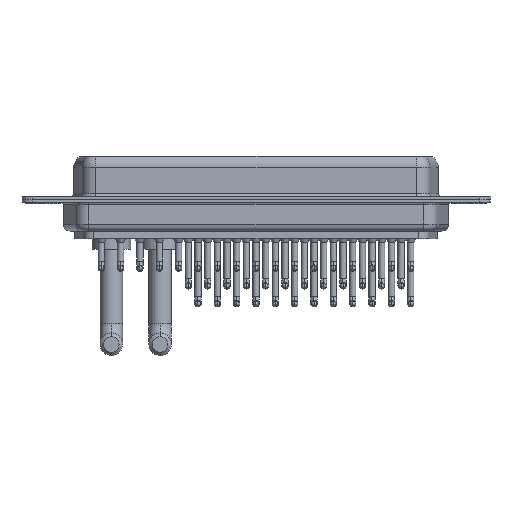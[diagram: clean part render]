
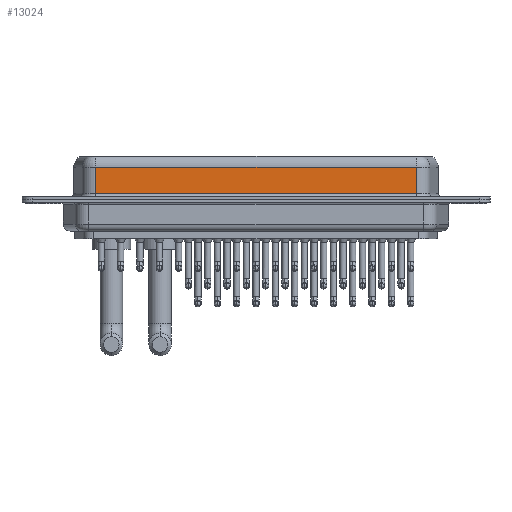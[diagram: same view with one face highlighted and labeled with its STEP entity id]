
A CAD part, front view. The second image highlights one B-rep face of the part: STEP entity #13024.
In plain terms, the highlighted planar face has unit normal (0, -1, 0).
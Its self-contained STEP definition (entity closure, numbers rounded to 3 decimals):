
#2371 = PLANE ( 'NONE',  #2853 ) ;
#2853 = AXIS2_PLACEMENT_3D ( 'NONE', #18748, #9419, #28192 ) ;
#3393 = ORIENTED_EDGE ( 'NONE', *, *, #6037, .T. ) ;
#5081 = DIRECTION ( 'NONE',  ( 0., 0., -1. ) ) ;
#5894 = VECTOR ( 'NONE', #27595, 1000. ) ;
#5993 = ORIENTED_EDGE ( 'NONE', *, *, #27063, .T. ) ;
#6037 = EDGE_CURVE ( 'NONE', #28539, #28702, #6899, .T. ) ;
#6092 = LINE ( 'NONE', #12981, #29181 ) ;
#6899 = LINE ( 'NONE', #8933, #15969 ) ;
#6987 = EDGE_CURVE ( 'NONE', #29571, #29864, #26237, .T. ) ;
#7423 = CARTESIAN_POINT ( 'NONE',  ( 53.41, -5.375, 6.4 ) ) ;
#8156 = CARTESIAN_POINT ( 'NONE',  ( 53.41, -5.375, 4.65 ) ) ;
#8422 = EDGE_LOOP ( 'NONE', ( #20438, #5993, #3393, #10921 ) ) ;
#8634 = LINE ( 'NONE', #15669, #5894 ) ;
#8933 = CARTESIAN_POINT ( 'NONE',  ( 7.59, -5.375, 6.4 ) ) ;
#9093 = CARTESIAN_POINT ( 'NONE',  ( 53.41, -5.375, 0.9 ) ) ;
#9419 = DIRECTION ( 'NONE',  ( 0., 1., 0. ) ) ;
#10921 = ORIENTED_EDGE ( 'NONE', *, *, #28016, .T. ) ;
#11266 = CARTESIAN_POINT ( 'NONE',  ( 7.59, -5.375, 4.65 ) ) ;
#11453 = FACE_OUTER_BOUND ( 'NONE', #8422, .T. ) ;
#11750 = DIRECTION ( 'NONE',  ( 0., 0., -1. ) ) ;
#12981 = CARTESIAN_POINT ( 'NONE',  ( 53.41, -5.375, 4.65 ) ) ;
#13024 = ADVANCED_FACE ( 'NONE', ( #11453 ), #2371, .F. ) ;
#15669 = CARTESIAN_POINT ( 'NONE',  ( 53.41, -5.375, 0.9 ) ) ;
#15969 = VECTOR ( 'NONE', #11750, 1000. ) ;
#18748 = CARTESIAN_POINT ( 'NONE',  ( 53.41, -5.375, 6.4 ) ) ;
#20438 = ORIENTED_EDGE ( 'NONE', *, *, #6987, .F. ) ;
#22236 = CARTESIAN_POINT ( 'NONE',  ( 7.59, -5.375, 0.9 ) ) ;
#24915 = VECTOR ( 'NONE', #5081, 1000. ) ;
#25070 = DIRECTION ( 'NONE',  ( -1., 0., 0. ) ) ;
#26237 = LINE ( 'NONE', #7423, #24915 ) ;
#27063 = EDGE_CURVE ( 'NONE', #29571, #28539, #6092, .T. ) ;
#27595 = DIRECTION ( 'NONE',  ( 1., 0., 0. ) ) ;
#28016 = EDGE_CURVE ( 'NONE', #28702, #29864, #8634, .T. ) ;
#28192 = DIRECTION ( 'NONE',  ( 0., 0., 1. ) ) ;
#28539 = VERTEX_POINT ( 'NONE', #11266 ) ;
#28702 = VERTEX_POINT ( 'NONE', #22236 ) ;
#29181 = VECTOR ( 'NONE', #25070, 1000. ) ;
#29571 = VERTEX_POINT ( 'NONE', #8156 ) ;
#29864 = VERTEX_POINT ( 'NONE', #9093 ) ;
